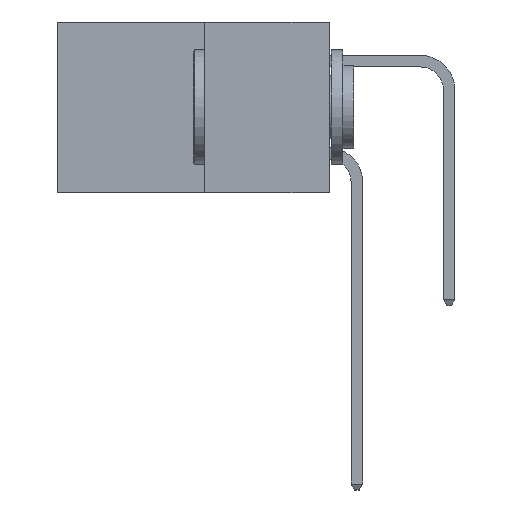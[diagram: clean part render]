
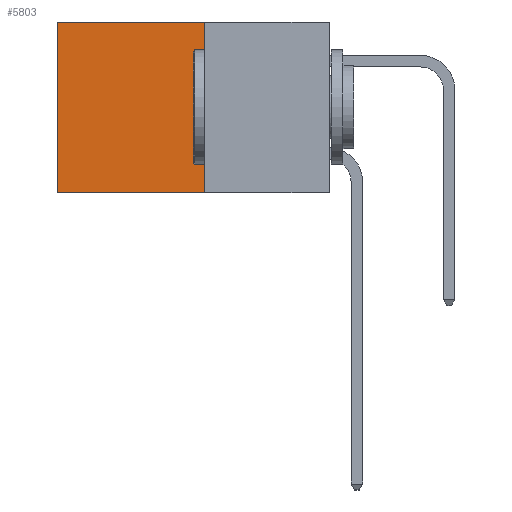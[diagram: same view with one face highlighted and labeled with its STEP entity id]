
A CAD part, left-side view. The second image highlights one B-rep face of the part: STEP entity #5803.
In plain terms, the highlighted planar face has unit normal (-1, 0, 0).
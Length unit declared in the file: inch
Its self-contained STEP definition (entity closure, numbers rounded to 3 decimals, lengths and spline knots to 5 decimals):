
#364 = EDGE_CURVE ( 'NONE', #14091, #9356, #2630, .T. ) ;
#887 = CARTESIAN_POINT ( 'NONE',  ( 0.277, 0.27, 0. ) ) ;
#1266 = CARTESIAN_POINT ( 'NONE',  ( 0.277, 0.59, 0. ) ) ;
#2130 = FACE_OUTER_BOUND ( 'NONE', #5466, .T. ) ;
#2630 = LINE ( 'NONE', #10347, #13685 ) ;
#2780 = CARTESIAN_POINT ( 'NONE',  ( 0.277, 0.59, -0.37 ) ) ;
#3661 = DIRECTION ( 'NONE',  ( 0., 0., -1. ) ) ;
#4285 = VERTEX_POINT ( 'NONE', #12424 ) ;
#5466 = EDGE_LOOP ( 'NONE', ( #7233, #13950, #16375, #6522 ) ) ;
#5474 = EDGE_CURVE ( 'NONE', #4285, #9356, #7207, .T. ) ;
#5799 = CARTESIAN_POINT ( 'NONE',  ( 0.277, 0.27, 0. ) ) ;
#5803 = ADVANCED_FACE ( 'NONE', ( #2130 ), #10306, .F. ) ;
#5855 = VECTOR ( 'NONE', #7268, 39.37008 ) ;
#6522 = ORIENTED_EDGE ( 'NONE', *, *, #16278, .T. ) ;
#6586 = CARTESIAN_POINT ( 'NONE',  ( 0.277, 0.27, -0.37 ) ) ;
#7207 = LINE ( 'NONE', #14264, #18019 ) ;
#7233 = ORIENTED_EDGE ( 'NONE', *, *, #364, .T. ) ;
#7268 = DIRECTION ( 'NONE',  ( 0., 1., 0. ) ) ;
#7505 = VERTEX_POINT ( 'NONE', #887 ) ;
#9356 = VERTEX_POINT ( 'NONE', #2780 ) ;
#9392 = LINE ( 'NONE', #6586, #13185 ) ;
#10142 = DIRECTION ( 'NONE',  ( 0., 0., -1. ) ) ;
#10165 = DIRECTION ( 'NONE',  ( 1., 0., 0. ) ) ;
#10306 = PLANE ( 'NONE',  #13192 ) ;
#10345 = CARTESIAN_POINT ( 'NONE',  ( 0.277, 0.27, -0.37 ) ) ;
#10347 = CARTESIAN_POINT ( 'NONE',  ( 0.277, 0.59, -0.37 ) ) ;
#12424 = CARTESIAN_POINT ( 'NONE',  ( 0.277, 0.27, -0.37 ) ) ;
#13185 = VECTOR ( 'NONE', #3661, 39.37008 ) ;
#13192 = AXIS2_PLACEMENT_3D ( 'NONE', #10345, #10165, #10142 ) ;
#13473 = LINE ( 'NONE', #5799, #5855 ) ;
#13685 = VECTOR ( 'NONE', #14934, 39.37008 ) ;
#13950 = ORIENTED_EDGE ( 'NONE', *, *, #5474, .F. ) ;
#14075 = DIRECTION ( 'NONE',  ( 0., 1., 0. ) ) ;
#14091 = VERTEX_POINT ( 'NONE', #1266 ) ;
#14264 = CARTESIAN_POINT ( 'NONE',  ( 0.277, 0.27, -0.37 ) ) ;
#14934 = DIRECTION ( 'NONE',  ( 0., 0., -1. ) ) ;
#16278 = EDGE_CURVE ( 'NONE', #7505, #14091, #13473, .T. ) ;
#16375 = ORIENTED_EDGE ( 'NONE', *, *, #18502, .F. ) ;
#18019 = VECTOR ( 'NONE', #14075, 39.37008 ) ;
#18502 = EDGE_CURVE ( 'NONE', #7505, #4285, #9392, .T. ) ;
